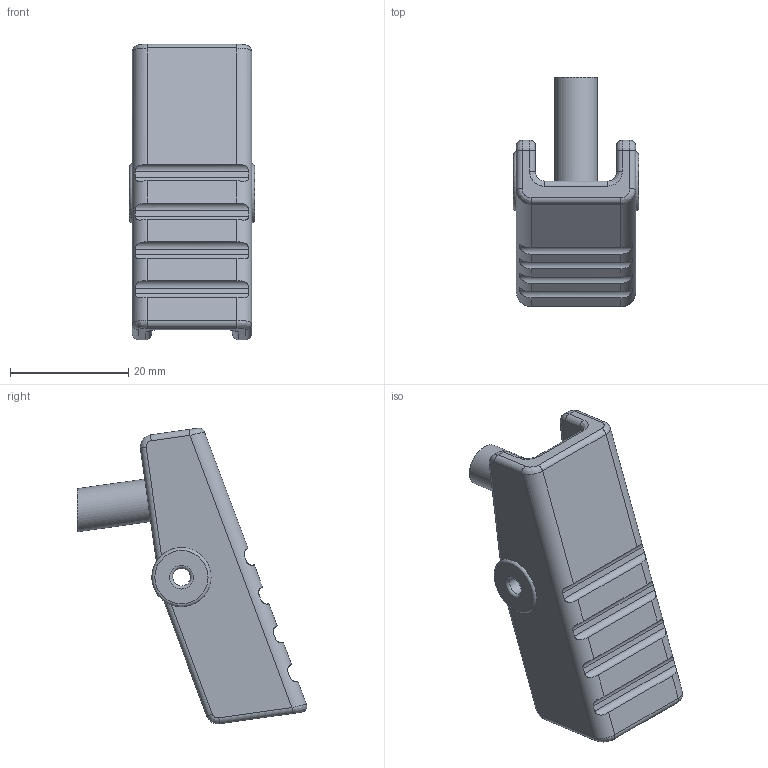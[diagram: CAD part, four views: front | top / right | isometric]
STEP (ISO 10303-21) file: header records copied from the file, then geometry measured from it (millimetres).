
FILE_DESCRIPTION(/* description */ (''),/* implementation_level */ '2;1');
FILE_NAME(/* name */ 'Custom Stock Latch.step',/* time_stamp */ '2022-05-27T20:30:35-05:00',/* author */ (''),/* organization */ (''),/* preprocessor_version */ 'ST-DEVELOPER v19',/* originating_system */ 'Autodesk Translation Framework v11.7.0.108',/* authorisation */ '');
FILE_SCHEMA (('AUTOMOTIVE_DESIGN { 1 0 10303 214 3 1 1 }'));
Length unit declared in the file: millimetre
Products named in the file (1): Custom Stock
Bounding box: 21.19 x 38.82 x 50.01 mm (x, y, z)
Volume: 8165.8 mm3; surface area: 5370.1 mm2
Topology: 1 solids, 1 shells, 88 faces, 212 edges, 128 vertices
Faces by surface type: cylinder 42, plane 24, bspline 16, torus 6
Full cylindrical faces by diameter (mm): 3 x2, 7.25 x1, 10 x1
Entity records: 3059 total; most frequent: CARTESIAN_POINT 989, DIRECTION 426, ORIENTED_EDGE 424, EDGE_CURVE 212, AXIS2_PLACEMENT_3D 165, VERTEX_POINT 128, LINE 96, VECTOR 96
